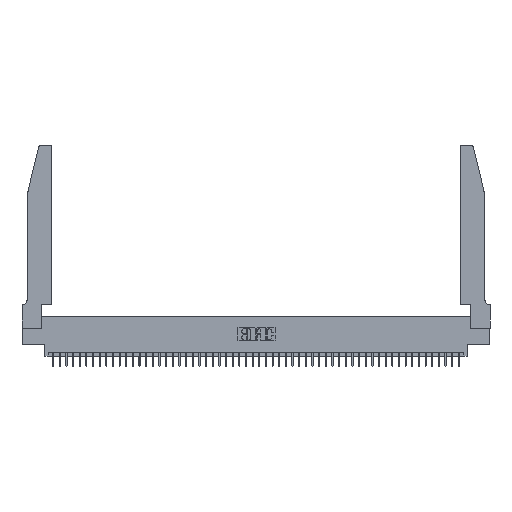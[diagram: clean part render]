
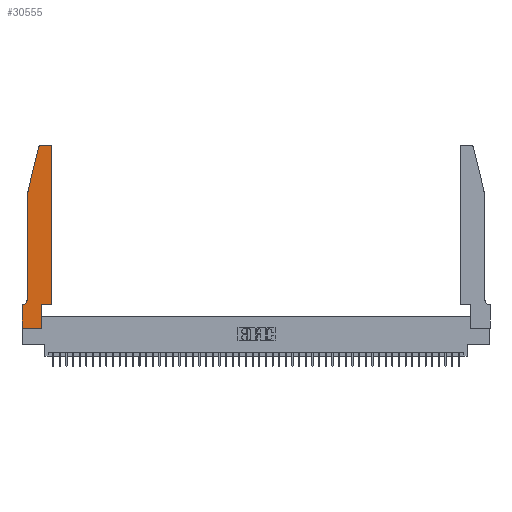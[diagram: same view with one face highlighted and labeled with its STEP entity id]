
A CAD part, top view. The second image highlights one B-rep face of the part: STEP entity #30555.
In plain terms, the highlighted planar face has unit normal (0, 0, 1).
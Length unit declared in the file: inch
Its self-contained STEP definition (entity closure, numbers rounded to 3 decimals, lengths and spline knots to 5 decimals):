
#416 = CARTESIAN_POINT ( 'NONE',  ( 0.4205, 2.75, 0.37 ) ) ;
#502 = DIRECTION ( 'NONE',  ( -1., 0., 0. ) ) ;
#1713 = LINE ( 'NONE', #31917, #24112 ) ;
#1766 = ORIENTED_EDGE ( 'NONE', *, *, #45258, .T. ) ;
#1770 = EDGE_CURVE ( 'NONE', #12745, #40525, #12645, .T. ) ;
#2637 = VERTEX_POINT ( 'NONE', #22421 ) ;
#3509 = CARTESIAN_POINT ( 'NONE',  ( 0., 0., 0.37 ) ) ;
#6597 = DIRECTION ( 'NONE',  ( -1., 0., 0. ) ) ;
#7210 = VECTOR ( 'NONE', #6597, 39.37008 ) ;
#7358 = ORIENTED_EDGE ( 'NONE', *, *, #42695, .T. ) ;
#7816 = VECTOR ( 'NONE', #35317, 39.37008 ) ;
#7978 = AXIS2_PLACEMENT_3D ( 'NONE', #34696, #11191, #38607 ) ;
#8476 = LINE ( 'NONE', #41826, #7210 ) ;
#8785 = EDGE_CURVE ( 'NONE', #48572, #24509, #43091, .T. ) ;
#9326 = ORIENTED_EDGE ( 'NONE', *, *, #16282, .T. ) ;
#9837 = ORIENTED_EDGE ( 'NONE', *, *, #21310, .T. ) ;
#9957 = CARTESIAN_POINT ( 'NONE',  ( 0.0755, 2., 0.37 ) ) ;
#11191 = DIRECTION ( 'NONE',  ( 0., 0., 1. ) ) ;
#12645 = CIRCLE ( 'NONE', #26112, 0.03 ) ;
#12738 = CARTESIAN_POINT ( 'NONE',  ( 0.0755, 0.35, 0.37 ) ) ;
#12745 = VERTEX_POINT ( 'NONE', #14156 ) ;
#13491 = DIRECTION ( 'NONE',  ( 1., 0., 0. ) ) ;
#13615 = LINE ( 'NONE', #26012, #21688 ) ;
#14074 = CARTESIAN_POINT ( 'NONE',  ( 0.0055, 0.35, 0.37 ) ) ;
#14156 = CARTESIAN_POINT ( 'NONE',  ( 0.284, 2.75, 0.37 ) ) ;
#15208 = EDGE_CURVE ( 'NONE', #2637, #26713, #13615, .T. ) ;
#16282 = EDGE_CURVE ( 'NONE', #20981, #48572, #16609, .T. ) ;
#16609 = LINE ( 'NONE', #12738, #36196 ) ;
#18527 = ORIENTED_EDGE ( 'NONE', *, *, #45041, .T. ) ;
#18626 = ORIENTED_EDGE ( 'NONE', *, *, #8785, .T. ) ;
#18910 = LINE ( 'NONE', #28237, #38482 ) ;
#19621 = LINE ( 'NONE', #31451, #7816 ) ;
#19861 = LINE ( 'NONE', #31857, #38092 ) ;
#20202 = VERTEX_POINT ( 'NONE', #36260 ) ;
#20981 = VERTEX_POINT ( 'NONE', #14074 ) ;
#21171 = DIRECTION ( 'NONE',  ( 0., 0., -1. ) ) ;
#21310 = EDGE_CURVE ( 'NONE', #47630, #33057, #1713, .T. ) ;
#21456 = CARTESIAN_POINT ( 'NONE',  ( 0.284, 2.72, 0.37 ) ) ;
#21688 = VECTOR ( 'NONE', #49332, 39.37008 ) ;
#21706 = ORIENTED_EDGE ( 'NONE', *, *, #34717, .T. ) ;
#22357 = VECTOR ( 'NONE', #29792, 39.37008 ) ;
#22421 = CARTESIAN_POINT ( 'NONE',  ( 0.2865, 0., 0.37 ) ) ;
#24082 = DIRECTION ( 'NONE',  ( 0., -1., 0. ) ) ;
#24112 = VECTOR ( 'NONE', #24082, 39.37008 ) ;
#24165 = ORIENTED_EDGE ( 'NONE', *, *, #15208, .T. ) ;
#24509 = VERTEX_POINT ( 'NONE', #35271 ) ;
#25381 = DIRECTION ( 'NONE',  ( 1., 0., 0. ) ) ;
#25855 = CARTESIAN_POINT ( 'NONE',  ( 0., 0., 0.37 ) ) ;
#26012 = CARTESIAN_POINT ( 'NONE',  ( 0.2865, 0.35, 0.37 ) ) ;
#26112 = AXIS2_PLACEMENT_3D ( 'NONE', #21456, #48708, #25381 ) ;
#26713 = VERTEX_POINT ( 'NONE', #39323 ) ;
#27387 = CIRCLE ( 'NONE', #41841, 0.07 ) ;
#28237 = CARTESIAN_POINT ( 'NONE',  ( 0.0755, 2., 0.37 ) ) ;
#28526 = LINE ( 'NONE', #3509, #48001 ) ;
#29030 = VERTEX_POINT ( 'NONE', #39121 ) ;
#29792 = DIRECTION ( 'NONE',  ( 0., -1., 0. ) ) ;
#30555 = ADVANCED_FACE ( 'NONE', ( #31308 ), #33076, .T. ) ;
#31308 = FACE_OUTER_BOUND ( 'NONE', #38074, .T. ) ;
#31451 = CARTESIAN_POINT ( 'NONE',  ( 0.4505, 0.35, 0.37 ) ) ;
#31857 = CARTESIAN_POINT ( 'NONE',  ( 0.4505, 0.35, 0.37 ) ) ;
#31917 = CARTESIAN_POINT ( 'NONE',  ( 0.0755, 2., 0.37 ) ) ;
#32139 = DIRECTION ( 'NONE',  ( -0.239, -0.971, 0. ) ) ;
#33057 = VERTEX_POINT ( 'NONE', #39313 ) ;
#33076 = PLANE ( 'NONE',  #36031 ) ;
#33655 = CARTESIAN_POINT ( 'NONE',  ( 0.25487, 2.72718, 0.37 ) ) ;
#34069 = VERTEX_POINT ( 'NONE', #416 ) ;
#34696 = CARTESIAN_POINT ( 'NONE',  ( 0.4205, 2.72, 0.37 ) ) ;
#34717 = EDGE_CURVE ( 'NONE', #29030, #20202, #19861, .T. ) ;
#35271 = CARTESIAN_POINT ( 'NONE',  ( 0., 0., 0.37 ) ) ;
#35317 = DIRECTION ( 'NONE',  ( 1., 0., 0. ) ) ;
#35394 = EDGE_CURVE ( 'NONE', #40525, #47630, #18910, .T. ) ;
#35677 = ORIENTED_EDGE ( 'NONE', *, *, #1770, .T. ) ;
#35764 = DIRECTION ( 'NONE',  ( 0., 1., 0. ) ) ;
#36031 = AXIS2_PLACEMENT_3D ( 'NONE', #48570, #36989, #13491 ) ;
#36196 = VECTOR ( 'NONE', #502, 39.37008 ) ;
#36260 = CARTESIAN_POINT ( 'NONE',  ( 0.4505, 2.72, 0.37 ) ) ;
#36957 = ORIENTED_EDGE ( 'NONE', *, *, #42013, .T. ) ;
#36989 = DIRECTION ( 'NONE',  ( 0., 0., 1. ) ) ;
#38074 = EDGE_LOOP ( 'NONE', ( #18527, #35677, #44840, #9837, #43128, #9326, #18626, #36957, #24165, #1766, #21706, #7358 ) ) ;
#38092 = VECTOR ( 'NONE', #35764, 39.37008 ) ;
#38482 = VECTOR ( 'NONE', #32139, 39.37008 ) ;
#38607 = DIRECTION ( 'NONE',  ( 1., 0., 0. ) ) ;
#39121 = CARTESIAN_POINT ( 'NONE',  ( 0.4505, 0.35, 0.37 ) ) ;
#39313 = CARTESIAN_POINT ( 'NONE',  ( 0.0755, 0.42, 0.37 ) ) ;
#39323 = CARTESIAN_POINT ( 'NONE',  ( 0.2865, 0.35, 0.37 ) ) ;
#40525 = VERTEX_POINT ( 'NONE', #33655 ) ;
#41061 = EDGE_CURVE ( 'NONE', #33057, #20981, #27387, .T. ) ;
#41826 = CARTESIAN_POINT ( 'NONE',  ( 0.2605, 2.75, 0.37 ) ) ;
#41841 = AXIS2_PLACEMENT_3D ( 'NONE', #44521, #21171, #48437 ) ;
#42013 = EDGE_CURVE ( 'NONE', #24509, #2637, #28526, .T. ) ;
#42036 = CARTESIAN_POINT ( 'NONE',  ( 0., 0.35, 0.37 ) ) ;
#42695 = EDGE_CURVE ( 'NONE', #20202, #34069, #50408, .T. ) ;
#43091 = LINE ( 'NONE', #25855, #22357 ) ;
#43128 = ORIENTED_EDGE ( 'NONE', *, *, #41061, .T. ) ;
#44521 = CARTESIAN_POINT ( 'NONE',  ( 0.0055, 0.42, 0.37 ) ) ;
#44840 = ORIENTED_EDGE ( 'NONE', *, *, #35394, .T. ) ;
#45041 = EDGE_CURVE ( 'NONE', #34069, #12745, #8476, .T. ) ;
#45258 = EDGE_CURVE ( 'NONE', #26713, #29030, #19621, .T. ) ;
#47630 = VERTEX_POINT ( 'NONE', #9957 ) ;
#48001 = VECTOR ( 'NONE', #50539, 39.37008 ) ;
#48437 = DIRECTION ( 'NONE',  ( -1., 0., 0. ) ) ;
#48570 = CARTESIAN_POINT ( 'NONE',  ( 0., 0.35, 0.37 ) ) ;
#48572 = VERTEX_POINT ( 'NONE', #42036 ) ;
#48708 = DIRECTION ( 'NONE',  ( 0., 0., 1. ) ) ;
#49332 = DIRECTION ( 'NONE',  ( 0., 1., 0. ) ) ;
#50408 = CIRCLE ( 'NONE', #7978, 0.03 ) ;
#50539 = DIRECTION ( 'NONE',  ( 1., 0., 0. ) ) ;
